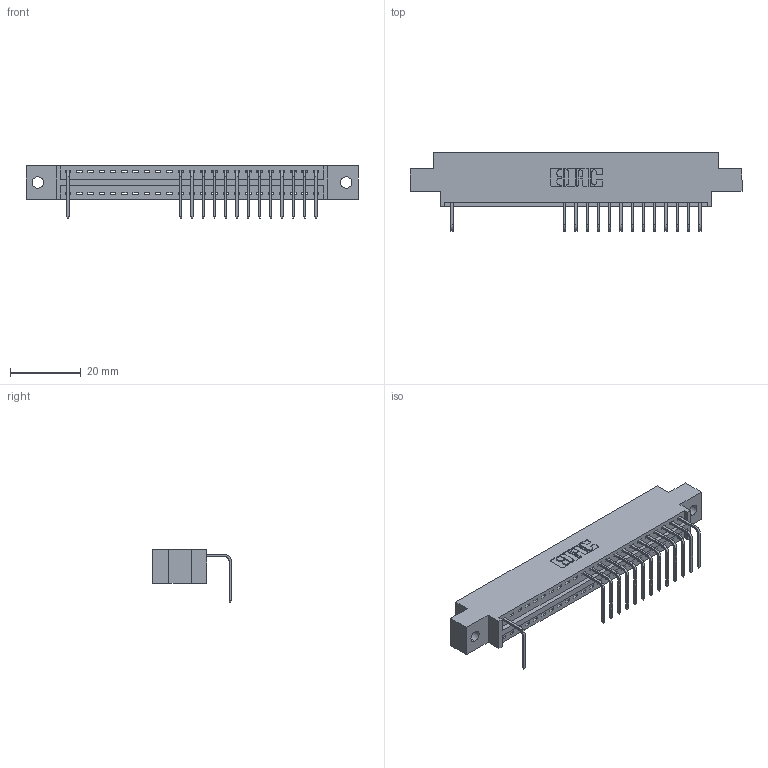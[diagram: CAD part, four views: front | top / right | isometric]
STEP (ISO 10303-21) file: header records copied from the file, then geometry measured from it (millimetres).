
FILE_DESCRIPTION (( 'STEP AP203' ), '1' );
FILE_NAME ('346-023-558-602.STEP', '2018-08-21T02:22:01', ( '' ), ( '' ), 'SwSTEP 2.0', 'SolidWorks 2016', '' );
FILE_SCHEMA (( 'CONFIG_CONTROL_DESIGN' ));
Length unit declared in the file: inch
Products named in the file (3): 346-023-558-602; 346 Part_0.170 Offset - 0.128 Dia; 345-292-001_558 Tail - 2
Assembly tree (15 placements, depth 2):
  346-023-558-602
    346 Part_0.170 Offset - 0.128 Dia
    345-292-001_558 Tail - 2  x14
Bounding box: 93.6 x 22.16 x 14.73 mm (x, y, z)
Volume: 8581 mm3; surface area: 10133.7 mm2
Topology: 15 solids, 15 shells, 1074 faces, 3267 edges, 2158 vertices
Faces by surface type: plane 758, cylinder 316
Entity records: 16763 total; most frequent: CARTESIAN_POINT 2928, ORIENTED_EDGE 2894, DIRECTION 2595, EDGE_CURVE 1447, VECTOR 1223, LINE 1223, VERTEX_POINT 962, AXIS2_PLACEMENT_3D 686
